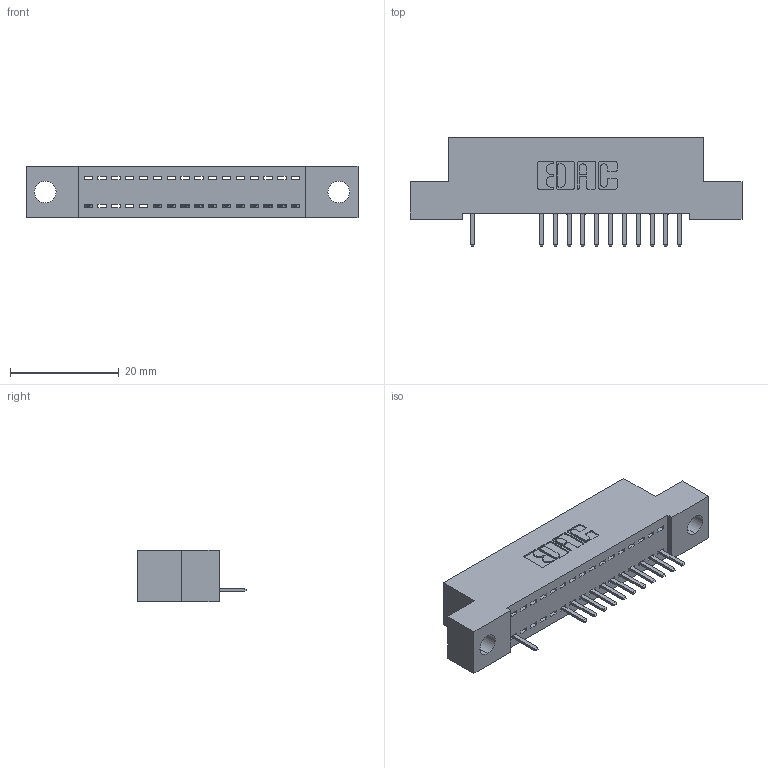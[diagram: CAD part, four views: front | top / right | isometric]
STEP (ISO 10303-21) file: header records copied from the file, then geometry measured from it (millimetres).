
FILE_DESCRIPTION (( 'STEP AP203' ), '1' );
FILE_NAME ('392-016-520-104.STEP', '2018-08-15T01:21:04', ( '' ), ( '' ), 'SwSTEP 2.0', 'SolidWorks 2016', '' );
FILE_SCHEMA (( 'CONFIG_CONTROL_DESIGN' ));
Length unit declared in the file: inch
Products named in the file (3): 342 Part_.156 TH; 345-292-001_345-293-120; 392-016-520-104
Assembly tree (13 placements, depth 2):
  392-016-520-104
    342 Part_.156 TH
    345-292-001_345-293-120  x12
Bounding box: 60.96 x 20.02 x 9.4 mm (x, y, z)
Volume: 5081.9 mm3; surface area: 6448.4 mm2
Topology: 13 solids, 13 shells, 902 faces, 2675 edges, 1750 vertices
Faces by surface type: plane 642, cylinder 260
Entity records: 13001 total; most frequent: CARTESIAN_POINT 2282, ORIENTED_EDGE 2226, DIRECTION 1961, EDGE_CURVE 1113, LINE 981, VECTOR 981, VERTEX_POINT 738, AXIS2_PLACEMENT_3D 490
